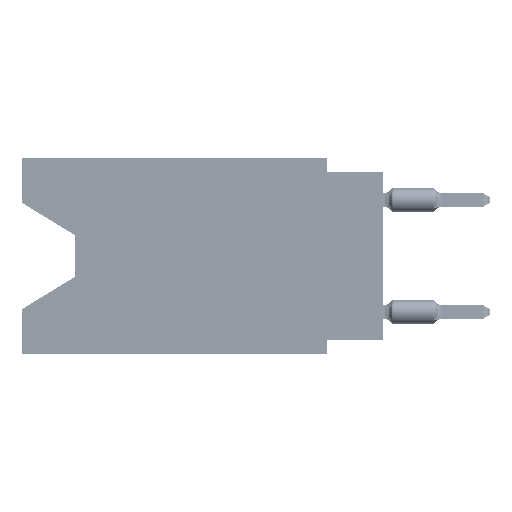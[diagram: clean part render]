
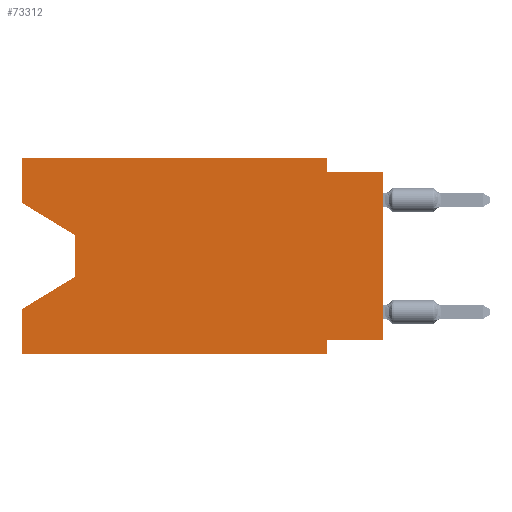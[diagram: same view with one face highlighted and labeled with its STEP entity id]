
A CAD part, left-side view. The second image highlights one B-rep face of the part: STEP entity #73312.
In plain terms, the highlighted planar face has unit normal (-1, 0, 0).
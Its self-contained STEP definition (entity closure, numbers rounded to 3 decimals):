
#2354 = EDGE_CURVE ( 'NONE', #34766, #76308, #93709, .T. ) ;
#2591 = EDGE_CURVE ( 'NONE', #19746, #76308, #38673, .T. ) ;
#2898 = CARTESIAN_POINT ( 'NONE',  ( 0., 16.383, -8.89 ) ) ;
#3903 = CARTESIAN_POINT ( 'NONE',  ( 0., 0., -0.635 ) ) ;
#5941 = VECTOR ( 'NONE', #46192, 1000. ) ;
#5981 = LINE ( 'NONE', #57928, #27993 ) ;
#7385 = VERTEX_POINT ( 'NONE', #112883 ) ;
#8123 = CARTESIAN_POINT ( 'NONE',  ( 0., 2.54, 0. ) ) ;
#8796 = VERTEX_POINT ( 'NONE', #47996 ) ;
#9391 = CARTESIAN_POINT ( 'NONE',  ( 0., 0., 0. ) ) ;
#12041 = ORIENTED_EDGE ( 'NONE', *, *, #89961, .F. ) ;
#13231 = VECTOR ( 'NONE', #31537, 1000. ) ;
#16244 = CARTESIAN_POINT ( 'NONE',  ( 0., 13.97, -5.385 ) ) ;
#16602 = ORIENTED_EDGE ( 'NONE', *, *, #93368, .F. ) ;
#16630 = ORIENTED_EDGE ( 'NONE', *, *, #22276, .T. ) ;
#17551 = LINE ( 'NONE', #87344, #38760 ) ;
#17968 = VERTEX_POINT ( 'NONE', #3903 ) ;
#18875 = VECTOR ( 'NONE', #84478, 1000. ) ;
#19746 = VERTEX_POINT ( 'NONE', #81460 ) ;
#20592 = ORIENTED_EDGE ( 'NONE', *, *, #2354, .T. ) ;
#21492 = LINE ( 'NONE', #101080, #85645 ) ;
#21803 = ORIENTED_EDGE ( 'NONE', *, *, #95753, .F. ) ;
#22276 = EDGE_CURVE ( 'NONE', #19746, #8796, #64073, .T. ) ;
#22830 = ORIENTED_EDGE ( 'NONE', *, *, #48054, .F. ) ;
#23080 = CARTESIAN_POINT ( 'NONE',  ( 0., 0., -8.255 ) ) ;
#24484 = ORIENTED_EDGE ( 'NONE', *, *, #2591, .F. ) ;
#26138 = DIRECTION ( 'NONE',  ( 0., 0., 1. ) ) ;
#27993 = VECTOR ( 'NONE', #31399, 1000. ) ;
#28010 = VERTEX_POINT ( 'NONE', #72674 ) ;
#28057 = CARTESIAN_POINT ( 'NONE',  ( 0., 16.383, 0. ) ) ;
#29268 = CARTESIAN_POINT ( 'NONE',  ( 0., 0., -0.635 ) ) ;
#30649 = AXIS2_PLACEMENT_3D ( 'NONE', #28057, #96734, #71897 ) ;
#31399 = DIRECTION ( 'NONE',  ( 0., -1., 0. ) ) ;
#31537 = DIRECTION ( 'NONE',  ( 0., -1., 0. ) ) ;
#32195 = VERTEX_POINT ( 'NONE', #8123 ) ;
#34513 = EDGE_CURVE ( 'NONE', #52786, #35177, #21492, .T. ) ;
#34766 = VERTEX_POINT ( 'NONE', #16244 ) ;
#35177 = VERTEX_POINT ( 'NONE', #82356 ) ;
#35377 = LINE ( 'NONE', #9391, #91166 ) ;
#36009 = DIRECTION ( 'NONE',  ( 0., 0., 1. ) ) ;
#36359 = DIRECTION ( 'NONE',  ( 0., 0., -1. ) ) ;
#38673 = LINE ( 'NONE', #46769, #5941 ) ;
#38760 = VECTOR ( 'NONE', #68915, 1000. ) ;
#40819 = ORIENTED_EDGE ( 'NONE', *, *, #34513, .T. ) ;
#45777 = LINE ( 'NONE', #88487, #78412 ) ;
#46192 = DIRECTION ( 'NONE',  ( 0., 0., 1. ) ) ;
#46769 = CARTESIAN_POINT ( 'NONE',  ( 0., 16.383, 0. ) ) ;
#46966 = VERTEX_POINT ( 'NONE', #112839 ) ;
#47996 = CARTESIAN_POINT ( 'NONE',  ( 0., 2.54, -8.89 ) ) ;
#48054 = EDGE_CURVE ( 'NONE', #52786, #28010, #45777, .T. ) ;
#48778 = CARTESIAN_POINT ( 'NONE',  ( 0., 2.54, -0.635 ) ) ;
#52786 = VERTEX_POINT ( 'NONE', #113149 ) ;
#56930 = LINE ( 'NONE', #29268, #13231 ) ;
#57928 = CARTESIAN_POINT ( 'NONE',  ( 0., 16.383, 0. ) ) ;
#59426 = ORIENTED_EDGE ( 'NONE', *, *, #77088, .T. ) ;
#62893 = CARTESIAN_POINT ( 'NONE',  ( 0., 13.97, -3.505 ) ) ;
#62930 = DIRECTION ( 'NONE',  ( 0., -1., 0. ) ) ;
#64073 = LINE ( 'NONE', #2898, #85368 ) ;
#65363 = DIRECTION ( 'NONE',  ( 0., 0., -1. ) ) ;
#67631 = CARTESIAN_POINT ( 'NONE',  ( 0., 2.54, -8.89 ) ) ;
#67689 = ORIENTED_EDGE ( 'NONE', *, *, #101317, .T. ) ;
#67827 = EDGE_CURVE ( 'NONE', #46966, #8796, #109182, .T. ) ;
#68915 = DIRECTION ( 'NONE',  ( 0., 0., -1. ) ) ;
#70630 = EDGE_LOOP ( 'NONE', ( #40819, #59426, #20592, #24484, #16630, #92881, #16602, #67689, #100834, #21803, #12041, #22830 ) ) ;
#71546 = VECTOR ( 'NONE', #100399, 1000. ) ;
#71776 = VERTEX_POINT ( 'NONE', #48778 ) ;
#71897 = DIRECTION ( 'NONE',  ( 0., 0., -1. ) ) ;
#72674 = CARTESIAN_POINT ( 'NONE',  ( 0., 16.383, 0. ) ) ;
#73312 = ADVANCED_FACE ( 'NONE', ( #79981 ), #114030, .F. ) ;
#73602 = VECTOR ( 'NONE', #36359, 1000. ) ;
#76308 = VERTEX_POINT ( 'NONE', #81582 ) ;
#77088 = EDGE_CURVE ( 'NONE', #35177, #34766, #106162, .T. ) ;
#78412 = VECTOR ( 'NONE', #36009, 1000. ) ;
#79981 = FACE_OUTER_BOUND ( 'NONE', #70630, .T. ) ;
#81460 = CARTESIAN_POINT ( 'NONE',  ( 0., 16.383, -8.89 ) ) ;
#81582 = CARTESIAN_POINT ( 'NONE',  ( 0., 16.383, -6.852 ) ) ;
#82356 = CARTESIAN_POINT ( 'NONE',  ( 0., 13.97, -3.505 ) ) ;
#83765 = DIRECTION ( 'NONE',  ( 0., -0.855, -0.519 ) ) ;
#84478 = DIRECTION ( 'NONE',  ( 0., 0.855, -0.519 ) ) ;
#85343 = LINE ( 'NONE', #23080, #71546 ) ;
#85368 = VECTOR ( 'NONE', #62930, 1000. ) ;
#85645 = VECTOR ( 'NONE', #83765, 1000. ) ;
#87344 = CARTESIAN_POINT ( 'NONE',  ( 0., 2.54, 0. ) ) ;
#88487 = CARTESIAN_POINT ( 'NONE',  ( 0., 16.383, 0. ) ) ;
#89961 = EDGE_CURVE ( 'NONE', #28010, #32195, #5981, .T. ) ;
#91166 = VECTOR ( 'NONE', #26138, 1000. ) ;
#92578 = CARTESIAN_POINT ( 'NONE',  ( 0., 13.97, -5.385 ) ) ;
#92881 = ORIENTED_EDGE ( 'NONE', *, *, #67827, .F. ) ;
#93368 = EDGE_CURVE ( 'NONE', #7385, #46966, #85343, .T. ) ;
#93709 = LINE ( 'NONE', #92578, #18875 ) ;
#95753 = EDGE_CURVE ( 'NONE', #32195, #71776, #17551, .T. ) ;
#96734 = DIRECTION ( 'NONE',  ( 1., 0., 0. ) ) ;
#100399 = DIRECTION ( 'NONE',  ( 0., 1., 0. ) ) ;
#100834 = ORIENTED_EDGE ( 'NONE', *, *, #107919, .F. ) ;
#101080 = CARTESIAN_POINT ( 'NONE',  ( 0., 16.383, -2.038 ) ) ;
#101317 = EDGE_CURVE ( 'NONE', #7385, #17968, #35377, .T. ) ;
#101673 = VECTOR ( 'NONE', #65363, 1000. ) ;
#106162 = LINE ( 'NONE', #62893, #73602 ) ;
#107919 = EDGE_CURVE ( 'NONE', #71776, #17968, #56930, .T. ) ;
#109182 = LINE ( 'NONE', #67631, #101673 ) ;
#112839 = CARTESIAN_POINT ( 'NONE',  ( 0., 2.54, -8.255 ) ) ;
#112883 = CARTESIAN_POINT ( 'NONE',  ( 0., 0., -8.255 ) ) ;
#113149 = CARTESIAN_POINT ( 'NONE',  ( 0., 16.383, -2.038 ) ) ;
#114030 = PLANE ( 'NONE',  #30649 ) ;
